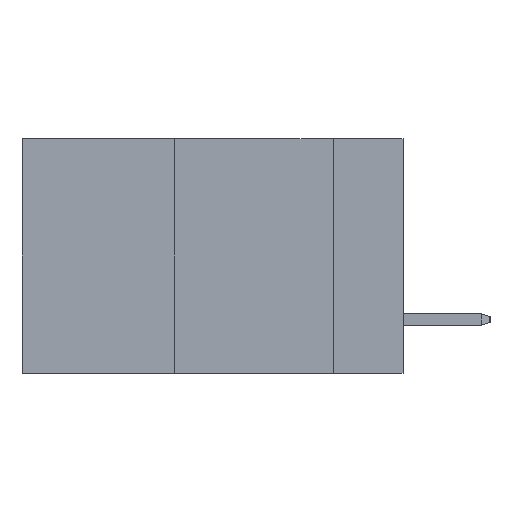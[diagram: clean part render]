
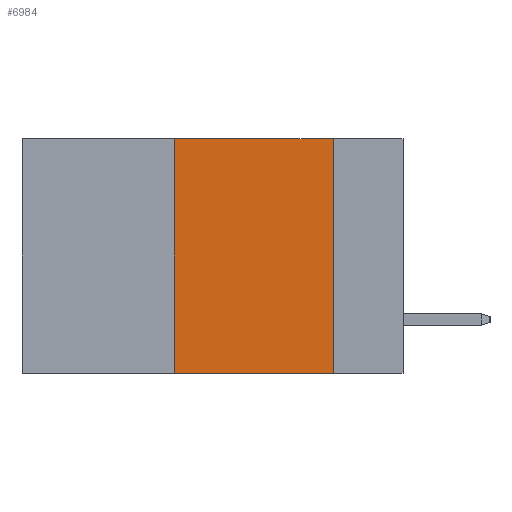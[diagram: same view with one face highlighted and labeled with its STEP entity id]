
A CAD part, left-side view. The second image highlights one B-rep face of the part: STEP entity #6984.
In plain terms, the highlighted planar face has unit normal (-1, 0, 0).
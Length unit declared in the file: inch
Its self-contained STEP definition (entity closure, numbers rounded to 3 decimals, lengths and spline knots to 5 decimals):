
#456 = VECTOR ( 'NONE', #3737, 39.37008 ) ;
#1148 = DIRECTION ( 'NONE',  ( 0., 0., -1. ) ) ;
#1254 = VERTEX_POINT ( 'NONE', #10944 ) ;
#1684 = VERTEX_POINT ( 'NONE', #6190 ) ;
#2147 = VECTOR ( 'NONE', #11340, 39.37008 ) ;
#2797 = PLANE ( 'NONE',  #11693 ) ;
#3054 = CARTESIAN_POINT ( 'NONE',  ( 0., 0.6, -0.37 ) ) ;
#3067 = VECTOR ( 'NONE', #11480, 39.37008 ) ;
#3683 = VERTEX_POINT ( 'NONE', #11169 ) ;
#3737 = DIRECTION ( 'NONE',  ( 0., 0., -1. ) ) ;
#3885 = LINE ( 'NONE', #7580, #3067 ) ;
#4494 = EDGE_CURVE ( 'NONE', #3683, #11639, #11315, .T. ) ;
#4649 = LINE ( 'NONE', #8539, #456 ) ;
#4896 = EDGE_CURVE ( 'NONE', #1684, #3683, #3885, .T. ) ;
#5032 = DIRECTION ( 'NONE',  ( 0., -1., 0. ) ) ;
#6190 = CARTESIAN_POINT ( 'NONE',  ( 0., 0.36, -0.37 ) ) ;
#6778 = CARTESIAN_POINT ( 'NONE',  ( 0., 0.6, 0. ) ) ;
#6984 = ADVANCED_FACE ( 'NONE', ( #9490 ), #2797, .F. ) ;
#7327 = VECTOR ( 'NONE', #5032, 39.37008 ) ;
#7580 = CARTESIAN_POINT ( 'NONE',  ( 0., 0.36, 0. ) ) ;
#7672 = DIRECTION ( 'NONE',  ( 1., 0., 0. ) ) ;
#7680 = LINE ( 'NONE', #3054, #2147 ) ;
#7796 = ORIENTED_EDGE ( 'NONE', *, *, #11679, .F. ) ;
#8271 = EDGE_CURVE ( 'NONE', #1684, #1254, #7680, .T. ) ;
#8539 = CARTESIAN_POINT ( 'NONE',  ( 0., 0.11, 0. ) ) ;
#8584 = CARTESIAN_POINT ( 'NONE',  ( 0., 0.6, 0. ) ) ;
#9452 = EDGE_LOOP ( 'NONE', ( #7796, #10818, #11674, #10201 ) ) ;
#9490 = FACE_OUTER_BOUND ( 'NONE', #9452, .T. ) ;
#10201 = ORIENTED_EDGE ( 'NONE', *, *, #8271, .T. ) ;
#10818 = ORIENTED_EDGE ( 'NONE', *, *, #4494, .F. ) ;
#10944 = CARTESIAN_POINT ( 'NONE',  ( 0., 0.11, -0.37 ) ) ;
#11169 = CARTESIAN_POINT ( 'NONE',  ( 0., 0.36, 0. ) ) ;
#11315 = LINE ( 'NONE', #6778, #7327 ) ;
#11340 = DIRECTION ( 'NONE',  ( 0., -1., 0. ) ) ;
#11345 = CARTESIAN_POINT ( 'NONE',  ( 0., 0.11, 0. ) ) ;
#11480 = DIRECTION ( 'NONE',  ( 0., 0., 1. ) ) ;
#11639 = VERTEX_POINT ( 'NONE', #11345 ) ;
#11674 = ORIENTED_EDGE ( 'NONE', *, *, #4896, .F. ) ;
#11679 = EDGE_CURVE ( 'NONE', #11639, #1254, #4649, .T. ) ;
#11693 = AXIS2_PLACEMENT_3D ( 'NONE', #8584, #7672, #1148 ) ;
